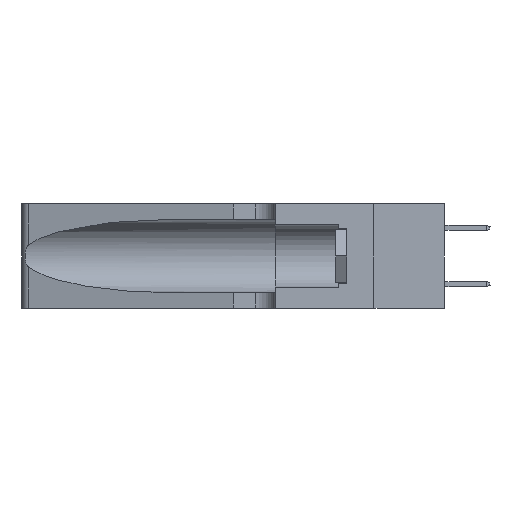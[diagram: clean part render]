
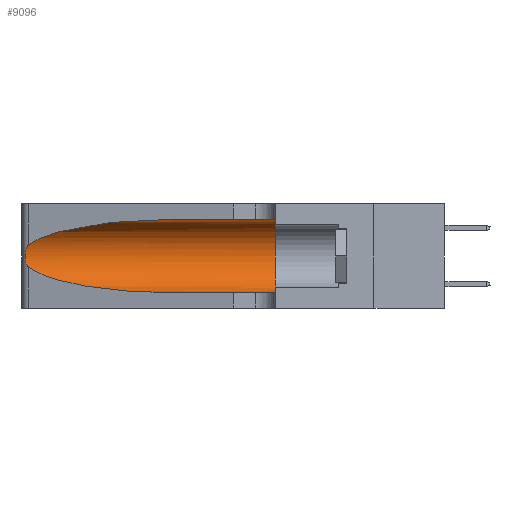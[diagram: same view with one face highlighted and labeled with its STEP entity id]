
A CAD part, left-side view. The second image highlights one B-rep face of the part: STEP entity #9096.
In plain terms, the highlighted cylindrical face has radius 3.308 mm (diameter 6.617 mm), a partial arc.
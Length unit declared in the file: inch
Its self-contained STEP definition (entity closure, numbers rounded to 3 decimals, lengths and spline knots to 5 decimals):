
#1262 = ORIENTED_EDGE ( 'NONE', *, *, #26553, .T. ) ;
#1735 = VECTOR ( 'NONE', #32198, 39.37008 ) ;
#2207 =( BOUNDED_CURVE ( )  B_SPLINE_CURVE ( 3, ( #30730, #33787, #13557, #31281 ),
 .UNSPECIFIED., .F., .F. ) 
 B_SPLINE_CURVE_WITH_KNOTS ( ( 4, 4 ),
 ( 1.5708, 2.84003 ),
 .UNSPECIFIED. ) 
 CURVE ( )  GEOMETRIC_REPRESENTATION_ITEM ( )  RATIONAL_B_SPLINE_CURVE ( ( 1., 0.87, 0.87, 1. ) ) 
 REPRESENTATION_ITEM ( '' )  );
#3409 = ORIENTED_EDGE ( 'NONE', *, *, #30278, .F. ) ;
#4136 = CARTESIAN_POINT ( 'NONE',  ( 0.25854, 1.2359, 0.20912 ) ) ;
#4154 = EDGE_LOOP ( 'NONE', ( #24895, #1262, #19599, #34591, #27523, #3409 ) ) ;
#4392 = CARTESIAN_POINT ( 'NONE',  ( 0.25487, 1.22718, 0.14631 ) ) ;
#5233 = CARTESIAN_POINT ( 'NONE',  ( 0.1305, 0.72297, 0.31525 ) ) ;
#5735 = LINE ( 'NONE', #36974, #36943 ) ;
#6954 = DIRECTION ( 'NONE',  ( 0., 1., 0. ) ) ;
#7143 = CARTESIAN_POINT ( 'NONE',  ( 0.26075, 1.23896, 0.178 ) ) ;
#7410 = CARTESIAN_POINT ( 'NONE',  ( 0.25787, 1.23484, 0.2124 ) ) ;
#9096 = ADVANCED_FACE ( 'NONE', ( #32477 ), #9294, .F. ) ;
#9294 = CYLINDRICAL_SURFACE ( 'NONE', #31467, 0.13025 ) ;
#9612 = VERTEX_POINT ( 'NONE', #37055 ) ;
#10187 = CARTESIAN_POINT ( 'NONE',  ( 0.26017, 1.23833, 0.17102 ) ) ;
#10427 = CARTESIAN_POINT ( 'NONE',  ( 0.25555, 1.22993, 0.14849 ) ) ;
#11040 = CARTESIAN_POINT ( 'NONE',  ( 0.1305, 1.61858, 0.05475 ) ) ;
#11295 = DIRECTION ( 'NONE',  ( 0., -1., 0. ) ) ;
#12011 = VERTEX_POINT ( 'NONE', #25757 ) ;
#12559 = LINE ( 'NONE', #11040, #1735 ) ;
#13050 = VERTEX_POINT ( 'NONE', #5233 ) ;
#13205 = CARTESIAN_POINT ( 'NONE',  ( 0.26018, 1.23835, 0.19895 ) ) ;
#13557 = CARTESIAN_POINT ( 'NONE',  ( 0.2373, 1.15595, 0.28018 ) ) ;
#14202 = CARTESIAN_POINT ( 'NONE',  ( 0.2373, 1.15595, 0.08982 ) ) ;
#14914 = EDGE_CURVE ( 'NONE', #13050, #12011, #2207, .T. ) ;
#16252 = CARTESIAN_POINT ( 'NONE',  ( 0.1305, 0.35, 0.05475 ) ) ;
#16423 = EDGE_CURVE ( 'NONE', #9612, #24214, #12559, .T. ) ;
#16459 = CARTESIAN_POINT ( 'NONE',  ( 0.1305, 0.35, 0.31525 ) ) ;
#17128 = VERTEX_POINT ( 'NONE', #16459 ) ;
#17248 = CARTESIAN_POINT ( 'NONE',  ( 0.18966, 0.96281, 0.05475 ) ) ;
#17504 = CARTESIAN_POINT ( 'NONE',  ( 0.1305, 0.72297, 0.05475 ) ) ;
#19599 = ORIENTED_EDGE ( 'NONE', *, *, #33838, .T. ) ;
#22211 = CARTESIAN_POINT ( 'NONE',  ( 0.25555, 1.22994, 0.2215 ) ) ;
#22477 = CARTESIAN_POINT ( 'NONE',  ( 0.25856, 1.23593, 0.16098 ) ) ;
#23471 = CARTESIAN_POINT ( 'NONE',  ( 0.25487, 1.22718, 0.14631 ) ) ;
#24214 = VERTEX_POINT ( 'NONE', #16252 ) ;
#24895 = ORIENTED_EDGE ( 'NONE', *, *, #14914, .T. ) ;
#25147 = EDGE_CURVE ( 'NONE', #17128, #24214, #35269, .T. ) ;
#25255 = CARTESIAN_POINT ( 'NONE',  ( 0.26075, 1.23896, 0.19203 ) ) ;
#25757 = CARTESIAN_POINT ( 'NONE',  ( 0.25487, 1.22718, 0.22369 ) ) ;
#26553 = EDGE_CURVE ( 'NONE', #12011, #38599, #31486, .T. ) ;
#26787 = CARTESIAN_POINT ( 'NONE',  ( 0.1305, 1.61858, 0.185 ) ) ;
#27523 = ORIENTED_EDGE ( 'NONE', *, *, #25147, .F. ) ;
#29737 = CARTESIAN_POINT ( 'NONE',  ( 0.25487, 1.22718, 0.14631 ) ) ;
#30278 = EDGE_CURVE ( 'NONE', #13050, #17128, #5735, .T. ) ;
#30730 = CARTESIAN_POINT ( 'NONE',  ( 0.1305, 0.72297, 0.31525 ) ) ;
#31003 = DIRECTION ( 'NONE',  ( 0., -1., 0. ) ) ;
#31137 = DIRECTION ( 'NONE',  ( 0., 0., 1. ) ) ;
#31281 = CARTESIAN_POINT ( 'NONE',  ( 0.25487, 1.22718, 0.22369 ) ) ;
#31323 = CARTESIAN_POINT ( 'NONE',  ( 0.25789, 1.23486, 0.15765 ) ) ;
#31467 = AXIS2_PLACEMENT_3D ( 'NONE', #26787, #11295, #32605 ) ;
#31486 = B_SPLINE_CURVE_WITH_KNOTS ( 'NONE', 3,
 ( #34225, #22211, #31578, #7410, #4136, #13205, #25255, #7143, #10187, #22477, #31323, #34363, #10427, #4392 ),
 .UNSPECIFIED., .F., .F.,
 ( 4, 2, 2, 2, 2, 2, 4 ),
 ( 0., 0.00027, 0.00053, 0.00107, 0.0016, 0.00187, 0.00214 ),
 .UNSPECIFIED. ) ;
#31578 = CARTESIAN_POINT ( 'NONE',  ( 0.25639, 1.23184, 0.21858 ) ) ;
#32198 = DIRECTION ( 'NONE',  ( 0., -1., 0. ) ) ;
#32477 = FACE_OUTER_BOUND ( 'NONE', #4154, .T. ) ;
#32605 = DIRECTION ( 'NONE',  ( 0., 0., -1. ) ) ;
#33787 = CARTESIAN_POINT ( 'NONE',  ( 0.18966, 0.96281, 0.31525 ) ) ;
#33838 = EDGE_CURVE ( 'NONE', #38599, #9612, #33867, .T. ) ;
#33867 =( BOUNDED_CURVE ( )  B_SPLINE_CURVE ( 3, ( #23471, #14202, #17248, #17504 ),
 .UNSPECIFIED., .F., .F. ) 
 B_SPLINE_CURVE_WITH_KNOTS ( ( 4, 4 ),
 ( 3.44316, 4.71239 ),
 .UNSPECIFIED. ) 
 CURVE ( )  GEOMETRIC_REPRESENTATION_ITEM ( )  RATIONAL_B_SPLINE_CURVE ( ( 1., 0.87, 0.87, 1. ) ) 
 REPRESENTATION_ITEM ( '' )  );
#33892 = CARTESIAN_POINT ( 'NONE',  ( 0.1305, 0.35, 0.185 ) ) ;
#34216 = AXIS2_PLACEMENT_3D ( 'NONE', #33892, #6954, #31137 ) ;
#34225 = CARTESIAN_POINT ( 'NONE',  ( 0.25487, 1.22718, 0.22369 ) ) ;
#34363 = CARTESIAN_POINT ( 'NONE',  ( 0.25639, 1.23186, 0.15144 ) ) ;
#34591 = ORIENTED_EDGE ( 'NONE', *, *, #16423, .T. ) ;
#35269 = CIRCLE ( 'NONE', #34216, 0.13025 ) ;
#36943 = VECTOR ( 'NONE', #31003, 39.37008 ) ;
#36974 = CARTESIAN_POINT ( 'NONE',  ( 0.1305, 1.61858, 0.31525 ) ) ;
#37055 = CARTESIAN_POINT ( 'NONE',  ( 0.1305, 0.72297, 0.05475 ) ) ;
#38599 = VERTEX_POINT ( 'NONE', #29737 ) ;
